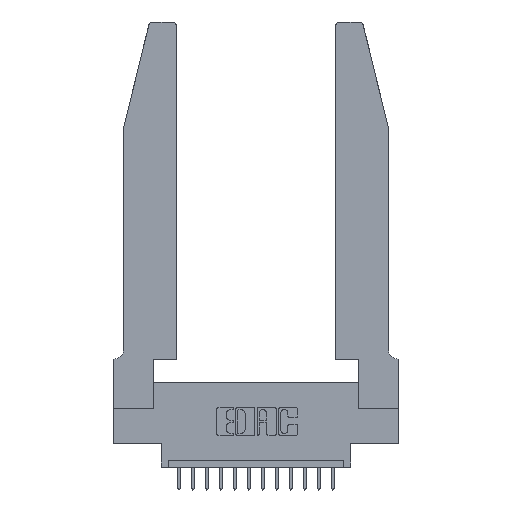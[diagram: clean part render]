
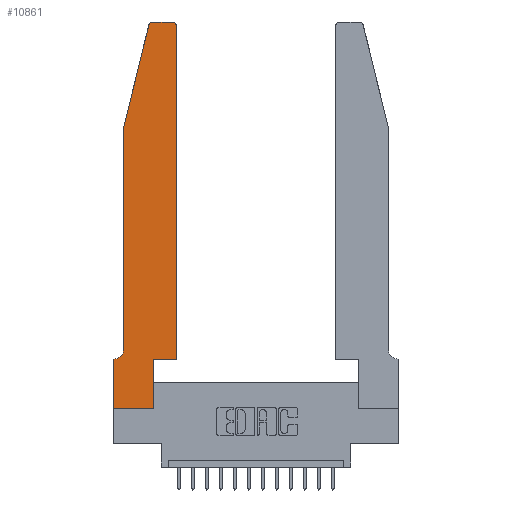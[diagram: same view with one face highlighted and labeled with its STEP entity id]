
A CAD part, top view. The second image highlights one B-rep face of the part: STEP entity #10861.
In plain terms, the highlighted planar face has unit normal (0, 0, 1).
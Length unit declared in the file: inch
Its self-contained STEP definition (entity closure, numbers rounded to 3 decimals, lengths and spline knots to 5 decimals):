
#319 = VERTEX_POINT ( 'NONE', #15043 ) ;
#408 = ORIENTED_EDGE ( 'NONE', *, *, #14096, .T. ) ;
#475 = CARTESIAN_POINT ( 'NONE',  ( 0., 0.35, 0.37 ) ) ;
#570 = LINE ( 'NONE', #14645, #3817 ) ;
#854 = EDGE_LOOP ( 'NONE', ( #4788, #2576, #5692, #11349, #7372, #4219, #15106, #15508, #408, #2659, #970, #1387 ) ) ;
#970 = ORIENTED_EDGE ( 'NONE', *, *, #5702, .T. ) ;
#1387 = ORIENTED_EDGE ( 'NONE', *, *, #17295, .T. ) ;
#1671 = VERTEX_POINT ( 'NONE', #16903 ) ;
#1876 = CARTESIAN_POINT ( 'NONE',  ( 0.25487, 2.72718, 0.37 ) ) ;
#2330 = VECTOR ( 'NONE', #11140, 39.37008 ) ;
#2433 = DIRECTION ( 'NONE',  ( 1., 0., 0. ) ) ;
#2474 = DIRECTION ( 'NONE',  ( 1., 0., 0. ) ) ;
#2576 = ORIENTED_EDGE ( 'NONE', *, *, #6480, .T. ) ;
#2599 = CARTESIAN_POINT ( 'NONE',  ( 0.4505, 0.35, 0.37 ) ) ;
#2617 = DIRECTION ( 'NONE',  ( 0., 0., 1. ) ) ;
#2659 = ORIENTED_EDGE ( 'NONE', *, *, #17706, .T. ) ;
#2906 = EDGE_CURVE ( 'NONE', #11095, #11452, #6761, .T. ) ;
#3185 = CARTESIAN_POINT ( 'NONE',  ( 0.0755, 2., 0.37 ) ) ;
#3334 = VECTOR ( 'NONE', #2433, 39.37008 ) ;
#3463 = DIRECTION ( 'NONE',  ( -1., 0., 0. ) ) ;
#3602 = DIRECTION ( 'NONE',  ( 0., 0., 1. ) ) ;
#3817 = VECTOR ( 'NONE', #3463, 39.37008 ) ;
#3964 = CARTESIAN_POINT ( 'NONE',  ( 0.0755, 2., 0.37 ) ) ;
#4219 = ORIENTED_EDGE ( 'NONE', *, *, #17353, .T. ) ;
#4475 = VERTEX_POINT ( 'NONE', #11346 ) ;
#4649 = LINE ( 'NONE', #2599, #13308 ) ;
#4698 = DIRECTION ( 'NONE',  ( 0., 0., -1. ) ) ;
#4788 = ORIENTED_EDGE ( 'NONE', *, *, #11212, .T. ) ;
#5071 = CARTESIAN_POINT ( 'NONE',  ( 0.0755, 0.42, 0.37 ) ) ;
#5281 = CIRCLE ( 'NONE', #16623, 0.03 ) ;
#5284 = AXIS2_PLACEMENT_3D ( 'NONE', #16821, #15410, #15459 ) ;
#5489 = VERTEX_POINT ( 'NONE', #475 ) ;
#5692 = ORIENTED_EDGE ( 'NONE', *, *, #16160, .T. ) ;
#5702 = EDGE_CURVE ( 'NONE', #10805, #5817, #10725, .T. ) ;
#5745 = PLANE ( 'NONE',  #5284 ) ;
#5817 = VERTEX_POINT ( 'NONE', #15274 ) ;
#6089 = DIRECTION ( 'NONE',  ( -1., 0., 0. ) ) ;
#6347 = CARTESIAN_POINT ( 'NONE',  ( 0.4205, 2.75, 0.37 ) ) ;
#6480 = EDGE_CURVE ( 'NONE', #10964, #10008, #5281, .T. ) ;
#6614 = VECTOR ( 'NONE', #16445, 39.37008 ) ;
#6700 = DIRECTION ( 'NONE',  ( 0., -1., 0. ) ) ;
#6761 = LINE ( 'NONE', #15214, #17414 ) ;
#6888 = DIRECTION ( 'NONE',  ( -1., 0., 0. ) ) ;
#7222 = CARTESIAN_POINT ( 'NONE',  ( 0.284, 2.75, 0.37 ) ) ;
#7372 = ORIENTED_EDGE ( 'NONE', *, *, #11658, .T. ) ;
#7494 = LINE ( 'NONE', #13656, #9189 ) ;
#8187 = LINE ( 'NONE', #3964, #9890 ) ;
#8237 = LINE ( 'NONE', #8614, #2330 ) ;
#8297 = DIRECTION ( 'NONE',  ( 0., -1., 0. ) ) ;
#8350 = LINE ( 'NONE', #10740, #3334 ) ;
#8614 = CARTESIAN_POINT ( 'NONE',  ( 0.2865, 0.35, 0.37 ) ) ;
#8817 = CIRCLE ( 'NONE', #15775, 0.07 ) ;
#8916 = CARTESIAN_POINT ( 'NONE',  ( 0.0055, 0.42, 0.37 ) ) ;
#9189 = VECTOR ( 'NONE', #6888, 39.37008 ) ;
#9890 = VECTOR ( 'NONE', #14978, 39.37008 ) ;
#10008 = VERTEX_POINT ( 'NONE', #1876 ) ;
#10066 = CIRCLE ( 'NONE', #17367, 0.03 ) ;
#10069 = EDGE_CURVE ( 'NONE', #5489, #4475, #12965, .T. ) ;
#10706 = VERTEX_POINT ( 'NONE', #16634 ) ;
#10725 = LINE ( 'NONE', #17814, #6614 ) ;
#10738 = CARTESIAN_POINT ( 'NONE',  ( 0., 0., 0.37 ) ) ;
#10740 = CARTESIAN_POINT ( 'NONE',  ( 0., 0., 0.37 ) ) ;
#10805 = VERTEX_POINT ( 'NONE', #15092 ) ;
#10861 = ADVANCED_FACE ( 'NONE', ( #16034 ), #5745, .T. ) ;
#10964 = VERTEX_POINT ( 'NONE', #7222 ) ;
#11095 = VERTEX_POINT ( 'NONE', #3185 ) ;
#11140 = DIRECTION ( 'NONE',  ( 0., 1., 0. ) ) ;
#11212 = EDGE_CURVE ( 'NONE', #16471, #10964, #570, .T. ) ;
#11346 = CARTESIAN_POINT ( 'NONE',  ( 0., 0., 0.37 ) ) ;
#11349 = ORIENTED_EDGE ( 'NONE', *, *, #2906, .T. ) ;
#11452 = VERTEX_POINT ( 'NONE', #5071 ) ;
#11658 = EDGE_CURVE ( 'NONE', #11452, #10706, #8817, .T. ) ;
#12442 = DIRECTION ( 'NONE',  ( 1., 0., 0. ) ) ;
#12965 = LINE ( 'NONE', #10738, #17356 ) ;
#13308 = VECTOR ( 'NONE', #2474, 39.37008 ) ;
#13656 = CARTESIAN_POINT ( 'NONE',  ( 0.0755, 0.35, 0.37 ) ) ;
#14096 = EDGE_CURVE ( 'NONE', #319, #1671, #8237, .T. ) ;
#14645 = CARTESIAN_POINT ( 'NONE',  ( 0.2605, 2.75, 0.37 ) ) ;
#14978 = DIRECTION ( 'NONE',  ( -0.239, -0.971, 0. ) ) ;
#15043 = CARTESIAN_POINT ( 'NONE',  ( 0.2865, 0., 0.37 ) ) ;
#15092 = CARTESIAN_POINT ( 'NONE',  ( 0.4505, 0.35, 0.37 ) ) ;
#15106 = ORIENTED_EDGE ( 'NONE', *, *, #10069, .T. ) ;
#15214 = CARTESIAN_POINT ( 'NONE',  ( 0.0755, 2., 0.37 ) ) ;
#15274 = CARTESIAN_POINT ( 'NONE',  ( 0.4505, 2.72, 0.37 ) ) ;
#15410 = DIRECTION ( 'NONE',  ( 0., 0., 1. ) ) ;
#15459 = DIRECTION ( 'NONE',  ( 1., 0., 0. ) ) ;
#15508 = ORIENTED_EDGE ( 'NONE', *, *, #17226, .T. ) ;
#15775 = AXIS2_PLACEMENT_3D ( 'NONE', #8916, #4698, #6089 ) ;
#16034 = FACE_OUTER_BOUND ( 'NONE', #854, .T. ) ;
#16090 = CARTESIAN_POINT ( 'NONE',  ( 0.284, 2.72, 0.37 ) ) ;
#16160 = EDGE_CURVE ( 'NONE', #10008, #11095, #8187, .T. ) ;
#16445 = DIRECTION ( 'NONE',  ( 0., 1., 0. ) ) ;
#16471 = VERTEX_POINT ( 'NONE', #6347 ) ;
#16623 = AXIS2_PLACEMENT_3D ( 'NONE', #16090, #3602, #17626 ) ;
#16634 = CARTESIAN_POINT ( 'NONE',  ( 0.0055, 0.35, 0.37 ) ) ;
#16821 = CARTESIAN_POINT ( 'NONE',  ( 0., 0.35, 0.37 ) ) ;
#16903 = CARTESIAN_POINT ( 'NONE',  ( 0.2865, 0.35, 0.37 ) ) ;
#17226 = EDGE_CURVE ( 'NONE', #4475, #319, #8350, .T. ) ;
#17295 = EDGE_CURVE ( 'NONE', #5817, #16471, #10066, .T. ) ;
#17353 = EDGE_CURVE ( 'NONE', #10706, #5489, #7494, .T. ) ;
#17356 = VECTOR ( 'NONE', #6700, 39.37008 ) ;
#17367 = AXIS2_PLACEMENT_3D ( 'NONE', #17958, #2617, #12442 ) ;
#17414 = VECTOR ( 'NONE', #8297, 39.37008 ) ;
#17626 = DIRECTION ( 'NONE',  ( 1., 0., 0. ) ) ;
#17706 = EDGE_CURVE ( 'NONE', #1671, #10805, #4649, .T. ) ;
#17814 = CARTESIAN_POINT ( 'NONE',  ( 0.4505, 0.35, 0.37 ) ) ;
#17958 = CARTESIAN_POINT ( 'NONE',  ( 0.4205, 2.72, 0.37 ) ) ;
